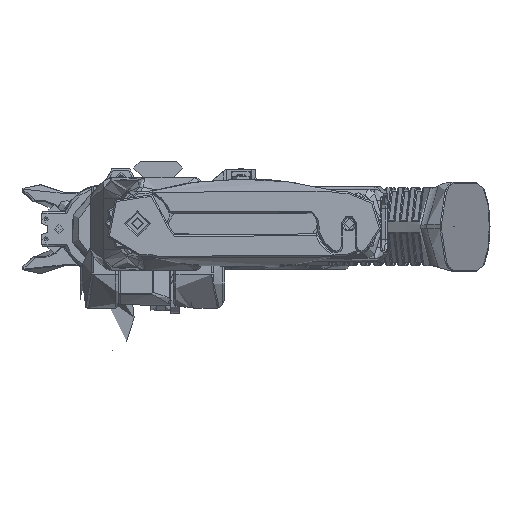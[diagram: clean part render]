
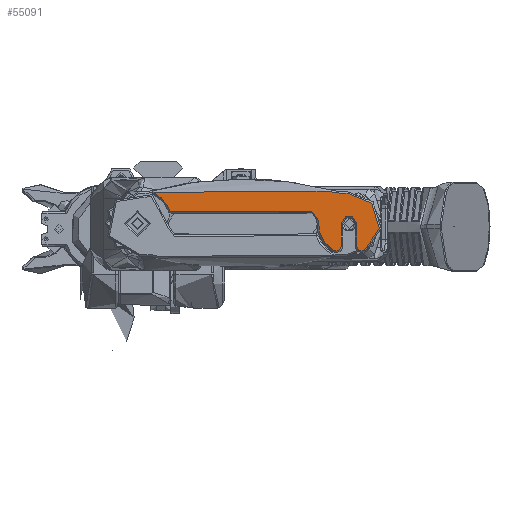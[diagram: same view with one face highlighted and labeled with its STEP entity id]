
A CAD part, left-side view. The second image highlights one B-rep face of the part: STEP entity #55091.
In plain terms, the highlighted planar face has unit normal (-1, 0, 0).
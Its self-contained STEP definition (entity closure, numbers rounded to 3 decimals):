
#3647=B_SPLINE_CURVE_WITH_KNOTS('',3,(#134436,#134437,#134438,#134439,#134440,
#134441,#134442),.UNSPECIFIED.,.F.,.F.,(4,1,1,1,4),(-2.302,-2.099,
-1.692,-1.285,-0.879),.UNSPECIFIED.);
#3649=B_SPLINE_CURVE_WITH_KNOTS('',3,(#134559,#134560,#134561,#134562,#134563),
 .UNSPECIFIED.,.F.,.F.,(4,1,4),(0.,0.189,
0.441),.UNSPECIFIED.);
#3650=B_SPLINE_CURVE_WITH_KNOTS('',3,(#134594,#134595,#134596,#134597,#134598,
#134599,#134600),.UNSPECIFIED.,.F.,.F.,(4,1,1,1,4),(-0.064,
-0.053,-0.047,-0.035,-0.024),
 .UNSPECIFIED.);
#5834=PLANE('',#59467);
#8684=FACE_OUTER_BOUND('',#12017,.T.);
#12017=EDGE_LOOP('',(#48666,#48667,#48668,#48669,#48670,#48671,#48672,#48673,
#48674,#48675,#48676,#48677,#48678,#48679));
#16471=LINE('',#134463,#20972);
#16475=LINE('',#134475,#20976);
#20972=VECTOR('',#71047,1000.);
#20976=VECTOR('',#71059,1000.);
#22847=CIRCLE('',#59437,15.733);
#22849=CIRCLE('',#59440,0.2);
#22851=CIRCLE('',#59444,25.8);
#22853=CIRCLE('',#59447,13.783);
#22855=CIRCLE('',#59450,2.2);
#22856=CIRCLE('',#59453,3.55);
#22859=CIRCLE('',#59458,2.2);
#22861=CIRCLE('',#59461,13.783);
#22862=CIRCLE('',#59462,0.2);
#27222=VERTEX_POINT('',#134390);
#27225=VERTEX_POINT('',#134395);
#27226=VERTEX_POINT('',#134399);
#27228=VERTEX_POINT('',#134432);
#27230=VERTEX_POINT('',#134444);
#27232=VERTEX_POINT('',#134450);
#27234=VERTEX_POINT('',#134456);
#27236=VERTEX_POINT('',#134462);
#27238=VERTEX_POINT('',#134468);
#27240=VERTEX_POINT('',#134474);
#27242=VERTEX_POINT('',#134480);
#27244=VERTEX_POINT('',#134486);
#27246=VERTEX_POINT('',#134526);
#27247=VERTEX_POINT('',#134592);
#34478=EDGE_CURVE('',#27225,#27222,#22847,.T.);
#34481=EDGE_CURVE('',#27222,#27226,#22849,.T.);
#34484=EDGE_CURVE('',#27226,#27228,#3647,.T.);
#34487=EDGE_CURVE('',#27228,#27230,#22851,.T.);
#34490=EDGE_CURVE('',#27230,#27232,#22853,.T.);
#34493=EDGE_CURVE('',#27232,#27234,#22855,.T.);
#34494=EDGE_CURVE('',#27234,#27236,#16471,.T.);
#34497=EDGE_CURVE('',#27236,#27238,#22856,.T.);
#34500=EDGE_CURVE('',#27238,#27240,#16475,.T.);
#34505=EDGE_CURVE('',#27240,#27242,#22859,.T.);
#34508=EDGE_CURVE('',#27242,#27244,#22861,.T.);
#34511=EDGE_CURVE('',#27244,#27246,#3649,.T.);
#34513=EDGE_CURVE('',#27246,#27247,#3650,.T.);
#34515=EDGE_CURVE('',#27247,#27225,#22862,.T.);
#48666=ORIENTED_EDGE('',*,*,#34478,.F.);
#48667=ORIENTED_EDGE('',*,*,#34515,.F.);
#48668=ORIENTED_EDGE('',*,*,#34513,.F.);
#48669=ORIENTED_EDGE('',*,*,#34511,.F.);
#48670=ORIENTED_EDGE('',*,*,#34508,.F.);
#48671=ORIENTED_EDGE('',*,*,#34505,.F.);
#48672=ORIENTED_EDGE('',*,*,#34500,.F.);
#48673=ORIENTED_EDGE('',*,*,#34497,.F.);
#48674=ORIENTED_EDGE('',*,*,#34494,.F.);
#48675=ORIENTED_EDGE('',*,*,#34493,.F.);
#48676=ORIENTED_EDGE('',*,*,#34490,.F.);
#48677=ORIENTED_EDGE('',*,*,#34487,.F.);
#48678=ORIENTED_EDGE('',*,*,#34484,.F.);
#48679=ORIENTED_EDGE('',*,*,#34481,.F.);
#55091=ADVANCED_FACE('',(#8684),#5834,.F.);
#59437=AXIS2_PLACEMENT_3D('',#134397,#71012,#71013);
#59440=AXIS2_PLACEMENT_3D('',#134403,#71019,#71020);
#59444=AXIS2_PLACEMENT_3D('',#134448,#71029,#71030);
#59447=AXIS2_PLACEMENT_3D('',#134454,#71036,#71037);
#59450=AXIS2_PLACEMENT_3D('',#134460,#71043,#71044);
#59453=AXIS2_PLACEMENT_3D('',#134469,#71052,#71053);
#59458=AXIS2_PLACEMENT_3D('',#134484,#71067,#71068);
#59461=AXIS2_PLACEMENT_3D('',#134490,#71074,#71075);
#59462=AXIS2_PLACEMENT_3D('',#134687,#71078,#71079);
#59467=AXIS2_PLACEMENT_3D('',#134718,#71094,#71095);
#71012=DIRECTION('center_axis',(-1.,0.,0.));
#71013=DIRECTION('ref_axis',(0.,0.,
1.));
#71019=DIRECTION('center_axis',(1.,0.,0.));
#71020=DIRECTION('ref_axis',(0.,0.994,0.108));
#71029=DIRECTION('center_axis',(-1.,0.,0.));
#71030=DIRECTION('ref_axis',(0.,0.102,-0.995));
#71036=DIRECTION('center_axis',(1.,0.,0.));
#71037=DIRECTION('ref_axis',(0.,0.,
1.));
#71043=DIRECTION('center_axis',(1.,0.,0.));
#71044=DIRECTION('ref_axis',(0.,0.502,-0.865));
#71047=DIRECTION('',(0.,0.,1.));
#71052=DIRECTION('center_axis',(-1.,0.,0.));
#71053=DIRECTION('ref_axis',(0.,0.,
1.));
#71059=DIRECTION('',(0.,0.,-1.));
#71067=DIRECTION('center_axis',(1.,0.,0.));
#71068=DIRECTION('ref_axis',(0.,-0.502,-0.865));
#71074=DIRECTION('center_axis',(1.,0.,0.));
#71075=DIRECTION('ref_axis',(0.,0.,
-1.));
#71078=DIRECTION('center_axis',(1.,0.,0.));
#71079=DIRECTION('ref_axis',(0.,0.938,-0.346));
#71094=DIRECTION('center_axis',(1.,0.,0.));
#71095=DIRECTION('ref_axis',(0.,0.,
-1.));
#134390=CARTESIAN_POINT('',(-464.681,17.032,14.558));
#134395=CARTESIAN_POINT('',(-464.681,9.906,6.251));
#134397=CARTESIAN_POINT('Origin',(-464.681,24.664,0.8));
#134399=CARTESIAN_POINT('',(-464.681,16.992,14.924));
#134403=CARTESIAN_POINT('Origin',(-464.681,16.935,14.733));
#134432=CARTESIAN_POINT('',(-464.681,-60.901,15.431));
#134436=CARTESIAN_POINT('Ctrl Pts',(-464.681,16.992,14.924));
#134437=CARTESIAN_POINT('Ctrl Pts',(-464.681,13.994,
15.82));
#134438=CARTESIAN_POINT('Ctrl Pts',(-464.681,4.163,
18.211));
#134439=CARTESIAN_POINT('Ctrl Pts',(-464.681,-15.408,
20.408));
#134440=CARTESIAN_POINT('Ctrl Pts',(-464.681,-40.121,
19.728));
#134441=CARTESIAN_POINT('Ctrl Pts',(-464.681,-54.695,
17.145));
#134442=CARTESIAN_POINT('Ctrl Pts',(-464.681,-60.901,
15.431));
#134444=CARTESIAN_POINT('',(-464.681,-69.442,14.554));
#134448=CARTESIAN_POINT('Origin',(-464.681,-67.769,40.3));
#134450=CARTESIAN_POINT('',(-464.681,-77.178,-11.164));
#134454=CARTESIAN_POINT('Origin',(-464.681,-70.336,0.8));
#134456=CARTESIAN_POINT('',(-464.681,-73.886,-9.254));
#134460=CARTESIAN_POINT('Origin',(-464.681,-76.086,-9.254));
#134462=CARTESIAN_POINT('',(-464.681,-73.886,0.8));
#134463=CARTESIAN_POINT('',(-464.681,-73.886,-4.2));
#134468=CARTESIAN_POINT('',(-464.681,-66.786,0.8));
#134469=CARTESIAN_POINT('Origin',(-464.681,-70.336,0.8));
#134474=CARTESIAN_POINT('',(-464.681,-66.786,-9.254));
#134475=CARTESIAN_POINT('',(-464.681,-66.786,-4.2));
#134480=CARTESIAN_POINT('',(-464.681,-63.494,-11.164));
#134484=CARTESIAN_POINT('Origin',(-464.681,-64.586,-9.254));
#134486=CARTESIAN_POINT('',(-464.681,-56.642,2.366));
#134490=CARTESIAN_POINT('Origin',(-464.681,-70.336,0.8));
#134526=CARTESIAN_POINT('',(-464.681,-53.692,6.508));
#134559=CARTESIAN_POINT('Ctrl Pts',(-464.681,-56.642,
2.366));
#134560=CARTESIAN_POINT('Ctrl Pts',(-464.681,-56.733,
3.159));
#134561=CARTESIAN_POINT('Ctrl Pts',(-464.681,-56.345,
5.071));
#134562=CARTESIAN_POINT('Ctrl Pts',(-464.681,-54.73,
6.277));
#134563=CARTESIAN_POINT('Ctrl Pts',(-464.681,-53.692,
6.508));
#134592=CARTESIAN_POINT('',(-464.681,9.671,6.126));
#134594=CARTESIAN_POINT('Ctrl Pts',(-464.681,-53.692,
6.508));
#134595=CARTESIAN_POINT('Ctrl Pts',(-464.681,-48.512,
7.659));
#134596=CARTESIAN_POINT('Ctrl Pts',(-464.681,-39.698,
8.977));
#134597=CARTESIAN_POINT('Ctrl Pts',(-464.681,-23.214,
9.829));
#134598=CARTESIAN_POINT('Ctrl Pts',(-464.681,-7.047,
9.222));
#134599=CARTESIAN_POINT('Ctrl Pts',(-464.681,4.531,
7.363));
#134600=CARTESIAN_POINT('Ctrl Pts',(-464.681,9.671,
6.126));
#134687=CARTESIAN_POINT('Origin',(-464.681,9.718,6.32));
#134718=CARTESIAN_POINT('Origin',(-464.681,-70.336,0.8));
